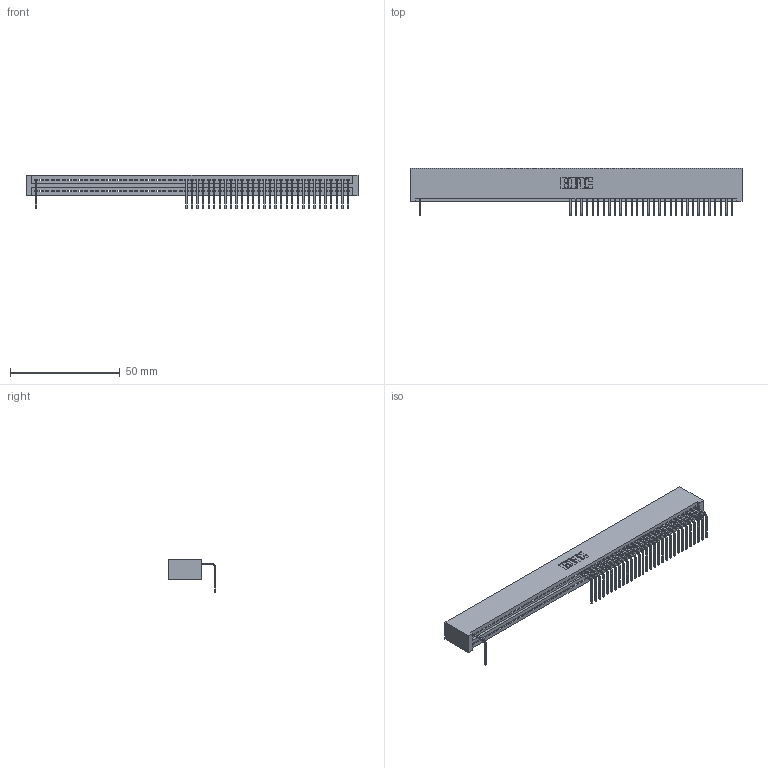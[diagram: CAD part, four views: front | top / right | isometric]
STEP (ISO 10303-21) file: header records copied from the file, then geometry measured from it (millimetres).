
FILE_DESCRIPTION (( 'STEP AP203' ), '1' );
FILE_NAME ('345-057-558-101.STEP', '2018-09-21T11:36:49', ( '' ), ( '' ), 'SwSTEP 2.0', 'SolidWorks 2016', '' );
FILE_SCHEMA (( 'CONFIG_CONTROL_DESIGN' ));
Length unit declared in the file: inch
Products named in the file (3): 345 Part_No Mounting Lugs; 345-292-001_558 Tail - 2; 345-057-558-101
Assembly tree (32 placements, depth 2):
  345-057-558-101
    345 Part_No Mounting Lugs
    345-292-001_558 Tail - 2  x31
Bounding box: 151.38 x 21.83 x 15.37 mm (x, y, z)
Volume: 14891.4 mm3; surface area: 19209.2 mm2
Topology: 32 solids, 32 shells, 2394 faces, 7363 edges, 4866 vertices
Faces by surface type: plane 1742, cylinder 652
Entity records: 39855 total; most frequent: ORIENTED_EDGE 7046, CARTESIAN_POINT 7029, DIRECTION 6081, EDGE_CURVE 3523, LINE 3171, VECTOR 3171, VERTEX_POINT 2346, AXIS2_PLACEMENT_3D 1455
